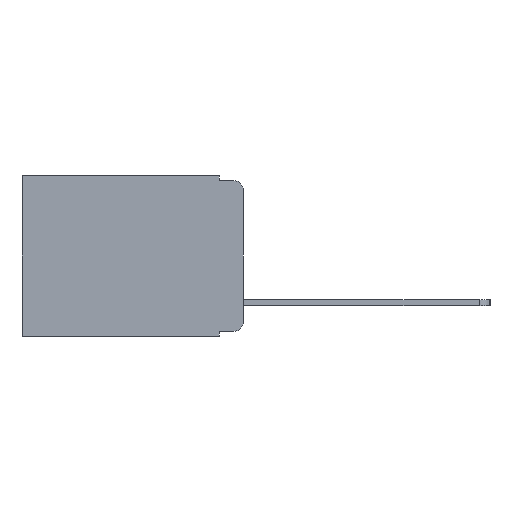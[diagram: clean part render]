
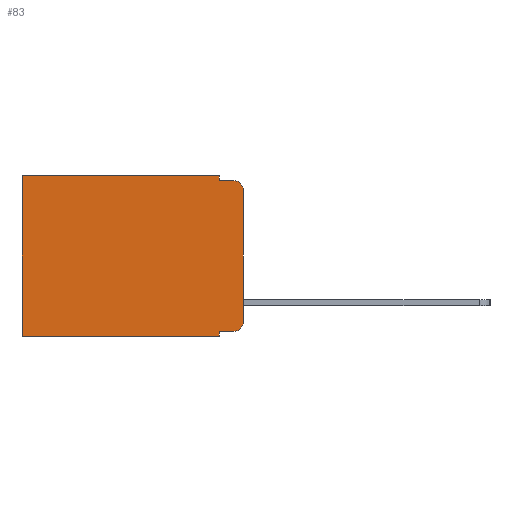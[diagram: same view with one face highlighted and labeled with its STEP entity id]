
A CAD part, left-side view. The second image highlights one B-rep face of the part: STEP entity #83.
In plain terms, the highlighted planar face has unit normal (-1, 0, 0).
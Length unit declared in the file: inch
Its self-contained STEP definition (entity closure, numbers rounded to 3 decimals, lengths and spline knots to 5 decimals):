
#83 = ADVANCED_FACE ( 'NONE', ( #11624 ), #7461, .F. ) ;
#331 = VERTEX_POINT ( 'NONE', #6757 ) ;
#504 = AXIS2_PLACEMENT_3D ( 'NONE', #9070, #22100, #10983 ) ;
#1685 = CARTESIAN_POINT ( 'NONE',  ( 0.298, 0., 0. ) ) ;
#2019 = VECTOR ( 'NONE', #9849, 39.37008 ) ;
#2203 = CARTESIAN_POINT ( 'NONE',  ( 0.298, 0.02, -0.01 ) ) ;
#2284 = VECTOR ( 'NONE', #18923, 39.37008 ) ;
#2993 = EDGE_CURVE ( 'NONE', #12914, #9850, #12949, .T. ) ;
#3359 = VERTEX_POINT ( 'NONE', #16683 ) ;
#3878 = ORIENTED_EDGE ( 'NONE', *, *, #9114, .F. ) ;
#3884 = ORIENTED_EDGE ( 'NONE', *, *, #9298, .F. ) ;
#4090 = EDGE_CURVE ( 'NONE', #17476, #3359, #17336, .T. ) ;
#4433 = VERTEX_POINT ( 'NONE', #14606 ) ;
#4650 = VECTOR ( 'NONE', #10166, 39.37008 ) ;
#4655 = DIRECTION ( 'NONE',  ( 0., 0., -1. ) ) ;
#4719 = CARTESIAN_POINT ( 'NONE',  ( 0.298, 0., 0. ) ) ;
#5073 = ORIENTED_EDGE ( 'NONE', *, *, #18741, .T. ) ;
#5183 = EDGE_CURVE ( 'NONE', #4433, #9850, #13058, .T. ) ;
#6517 = AXIS2_PLACEMENT_3D ( 'NONE', #4719, #6940, #4655 ) ;
#6757 = CARTESIAN_POINT ( 'NONE',  ( 0.298, 0., -0.313 ) ) ;
#6834 = VERTEX_POINT ( 'NONE', #22241 ) ;
#6940 = DIRECTION ( 'NONE',  ( 1., 0., 0. ) ) ;
#7198 = VECTOR ( 'NONE', #18278, 39.37008 ) ;
#7461 = PLANE ( 'NONE',  #6517 ) ;
#7507 = LINE ( 'NONE', #1685, #2284 ) ;
#7528 = EDGE_LOOP ( 'NONE', ( #3884, #15581, #7854, #21854, #5073, #15305, #17885, #3878, #12590, #12300 ) ) ;
#7854 = ORIENTED_EDGE ( 'NONE', *, *, #19158, .F. ) ;
#7988 = VECTOR ( 'NONE', #13956, 39.37008 ) ;
#8149 = CIRCLE ( 'NONE', #18487, 0.02 ) ;
#8407 = EDGE_CURVE ( 'NONE', #19355, #331, #8149, .T. ) ;
#8643 = VECTOR ( 'NONE', #20353, 39.37008 ) ;
#8922 = EDGE_CURVE ( 'NONE', #21755, #19355, #11429, .T. ) ;
#9070 = CARTESIAN_POINT ( 'NONE',  ( 0.298, 0.02, -0.03 ) ) ;
#9114 = EDGE_CURVE ( 'NONE', #21755, #12914, #12881, .T. ) ;
#9138 = DIRECTION ( 'NONE',  ( 0., 1., 0. ) ) ;
#9298 = EDGE_CURVE ( 'NONE', #6834, #331, #7507, .T. ) ;
#9299 = CARTESIAN_POINT ( 'NONE',  ( 0.298, 0.051, -0.333 ) ) ;
#9761 = CARTESIAN_POINT ( 'NONE',  ( 0.298, 0.051, 0. ) ) ;
#9838 = LINE ( 'NONE', #21327, #4650 ) ;
#9849 = DIRECTION ( 'NONE',  ( 0., 0., -1. ) ) ;
#9850 = VERTEX_POINT ( 'NONE', #11102 ) ;
#10166 = DIRECTION ( 'NONE',  ( 0., -1., 0. ) ) ;
#10671 = CARTESIAN_POINT ( 'NONE',  ( 0.298, 0.02, -0.313 ) ) ;
#10983 = DIRECTION ( 'NONE',  ( 0., 0., -1. ) ) ;
#11102 = CARTESIAN_POINT ( 'NONE',  ( 0.298, 0.473, -0.343 ) ) ;
#11429 = LINE ( 'NONE', #21385, #20727 ) ;
#11624 = FACE_OUTER_BOUND ( 'NONE', #7528, .T. ) ;
#12300 = ORIENTED_EDGE ( 'NONE', *, *, #8407, .T. ) ;
#12571 = DIRECTION ( 'NONE',  ( 0., 0., -1. ) ) ;
#12590 = ORIENTED_EDGE ( 'NONE', *, *, #8922, .T. ) ;
#12881 = LINE ( 'NONE', #23636, #7198 ) ;
#12914 = VERTEX_POINT ( 'NONE', #22634 ) ;
#12949 = LINE ( 'NONE', #14317, #16755 ) ;
#13058 = LINE ( 'NONE', #15769, #7988 ) ;
#13729 = LINE ( 'NONE', #20279, #8643 ) ;
#13956 = DIRECTION ( 'NONE',  ( 0., 0., -1. ) ) ;
#14304 = CIRCLE ( 'NONE', #504, 0.02 ) ;
#14317 = CARTESIAN_POINT ( 'NONE',  ( 0.298, 0., -0.343 ) ) ;
#14606 = CARTESIAN_POINT ( 'NONE',  ( 0.298, 0.473, 0. ) ) ;
#15265 = VERTEX_POINT ( 'NONE', #2203 ) ;
#15305 = ORIENTED_EDGE ( 'NONE', *, *, #5183, .T. ) ;
#15581 = ORIENTED_EDGE ( 'NONE', *, *, #18717, .T. ) ;
#15769 = CARTESIAN_POINT ( 'NONE',  ( 0.298, 0.473, 0. ) ) ;
#16683 = CARTESIAN_POINT ( 'NONE',  ( 0.298, 0.051, -0.01 ) ) ;
#16755 = VECTOR ( 'NONE', #9138, 39.37008 ) ;
#17336 = LINE ( 'NONE', #9761, #2019 ) ;
#17476 = VERTEX_POINT ( 'NONE', #23787 ) ;
#17885 = ORIENTED_EDGE ( 'NONE', *, *, #2993, .F. ) ;
#18278 = DIRECTION ( 'NONE',  ( 0., 0., -1. ) ) ;
#18487 = AXIS2_PLACEMENT_3D ( 'NONE', #10671, #23595, #12571 ) ;
#18717 = EDGE_CURVE ( 'NONE', #6834, #15265, #14304, .T. ) ;
#18741 = EDGE_CURVE ( 'NONE', #17476, #4433, #13729, .T. ) ;
#18923 = DIRECTION ( 'NONE',  ( 0., 0., -1. ) ) ;
#19158 = EDGE_CURVE ( 'NONE', #3359, #15265, #9838, .T. ) ;
#19355 = VERTEX_POINT ( 'NONE', #20123 ) ;
#20123 = CARTESIAN_POINT ( 'NONE',  ( 0.298, 0.02, -0.333 ) ) ;
#20279 = CARTESIAN_POINT ( 'NONE',  ( 0.298, 0., 0. ) ) ;
#20353 = DIRECTION ( 'NONE',  ( 0., 1., 0. ) ) ;
#20727 = VECTOR ( 'NONE', #23182, 39.37008 ) ;
#21327 = CARTESIAN_POINT ( 'NONE',  ( 0.298, 0.051, -0.01 ) ) ;
#21385 = CARTESIAN_POINT ( 'NONE',  ( 0.298, 0.051, -0.333 ) ) ;
#21755 = VERTEX_POINT ( 'NONE', #9299 ) ;
#21854 = ORIENTED_EDGE ( 'NONE', *, *, #4090, .F. ) ;
#22100 = DIRECTION ( 'NONE',  ( -1., 0., 0. ) ) ;
#22241 = CARTESIAN_POINT ( 'NONE',  ( 0.298, 0., -0.03 ) ) ;
#22634 = CARTESIAN_POINT ( 'NONE',  ( 0.298, 0.051, -0.343 ) ) ;
#23182 = DIRECTION ( 'NONE',  ( 0., -1., 0. ) ) ;
#23595 = DIRECTION ( 'NONE',  ( -1., 0., 0. ) ) ;
#23636 = CARTESIAN_POINT ( 'NONE',  ( 0.298, 0.051, 0. ) ) ;
#23787 = CARTESIAN_POINT ( 'NONE',  ( 0.298, 0.051, 0. ) ) ;
